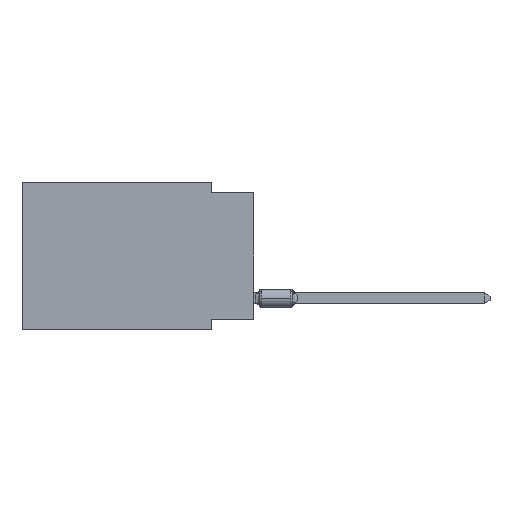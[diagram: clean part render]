
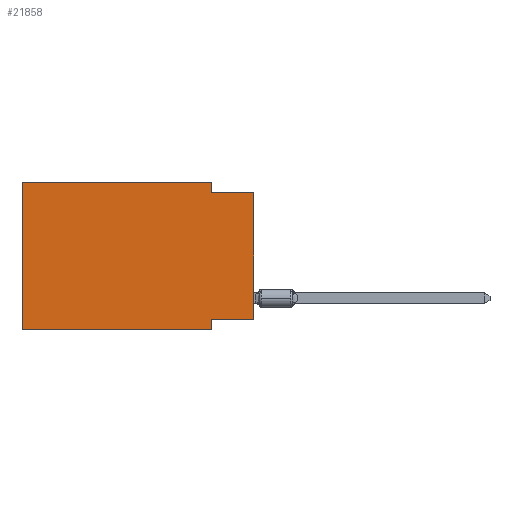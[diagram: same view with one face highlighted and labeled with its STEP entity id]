
A CAD part, left-side view. The second image highlights one B-rep face of the part: STEP entity #21858.
In plain terms, the highlighted planar face has unit normal (-1, 0, 0).
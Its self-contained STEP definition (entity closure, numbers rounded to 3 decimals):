
#670 = EDGE_LOOP ( 'NONE', ( #10321, #4042, #5680, #9196, #29071, #11287, #16565, #27068 ) ) ;
#789 = VECTOR ( 'NONE', #19286, 1000. ) ;
#1249 = CARTESIAN_POINT ( 'NONE',  ( 0., 2.54, -0.635 ) ) ;
#1926 = CARTESIAN_POINT ( 'NONE',  ( 0., 0., -0.635 ) ) ;
#3146 = CARTESIAN_POINT ( 'NONE',  ( 0., 0., 0. ) ) ;
#3660 = VECTOR ( 'NONE', #11100, 1000. ) ;
#4042 = ORIENTED_EDGE ( 'NONE', *, *, #23604, .F. ) ;
#4659 = VECTOR ( 'NONE', #29350, 1000. ) ;
#4697 = LINE ( 'NONE', #21197, #24072 ) ;
#5151 = VECTOR ( 'NONE', #9978, 1000. ) ;
#5238 = AXIS2_PLACEMENT_3D ( 'NONE', #20016, #29254, #8514 ) ;
#5680 = ORIENTED_EDGE ( 'NONE', *, *, #18365, .F. ) ;
#6106 = LINE ( 'NONE', #15334, #23554 ) ;
#7265 = DIRECTION ( 'NONE',  ( 0., 0., 1. ) ) ;
#7294 = VERTEX_POINT ( 'NONE', #9585 ) ;
#7629 = CARTESIAN_POINT ( 'NONE',  ( 0., 2.54, 0. ) ) ;
#7830 = VECTOR ( 'NONE', #20546, 1000. ) ;
#8514 = DIRECTION ( 'NONE',  ( 0., 0., -1. ) ) ;
#9196 = ORIENTED_EDGE ( 'NONE', *, *, #9801, .F. ) ;
#9410 = CARTESIAN_POINT ( 'NONE',  ( 0., 13.97, -8.89 ) ) ;
#9551 = DIRECTION ( 'NONE',  ( 0., 0., -1. ) ) ;
#9585 = CARTESIAN_POINT ( 'NONE',  ( 0., 2.54, -8.255 ) ) ;
#9686 = CARTESIAN_POINT ( 'NONE',  ( 0., 0., -0.635 ) ) ;
#9801 = EDGE_CURVE ( 'NONE', #24391, #15032, #28203, .T. ) ;
#9978 = DIRECTION ( 'NONE',  ( 0., -1., 0. ) ) ;
#10321 = ORIENTED_EDGE ( 'NONE', *, *, #23571, .T. ) ;
#11100 = DIRECTION ( 'NONE',  ( 0., -1., 0. ) ) ;
#11287 = ORIENTED_EDGE ( 'NONE', *, *, #15395, .T. ) ;
#11358 = EDGE_CURVE ( 'NONE', #7294, #27699, #4697, .T. ) ;
#13210 = CARTESIAN_POINT ( 'NONE',  ( 0., 13.97, -8.89 ) ) ;
#15032 = VERTEX_POINT ( 'NONE', #17481 ) ;
#15334 = CARTESIAN_POINT ( 'NONE',  ( 0., 13.97, 0. ) ) ;
#15395 = EDGE_CURVE ( 'NONE', #28291, #27699, #22596, .T. ) ;
#15564 = LINE ( 'NONE', #15872, #4659 ) ;
#15872 = CARTESIAN_POINT ( 'NONE',  ( 0., 0., -8.255 ) ) ;
#16565 = ORIENTED_EDGE ( 'NONE', *, *, #11358, .F. ) ;
#16592 = EDGE_CURVE ( 'NONE', #28291, #24391, #6106, .T. ) ;
#17481 = CARTESIAN_POINT ( 'NONE',  ( 0., 2.54, 0. ) ) ;
#17540 = VERTEX_POINT ( 'NONE', #1926 ) ;
#18365 = EDGE_CURVE ( 'NONE', #15032, #18476, #18839, .T. ) ;
#18418 = CARTESIAN_POINT ( 'NONE',  ( 0., 13.97, 0. ) ) ;
#18476 = VERTEX_POINT ( 'NONE', #1249 ) ;
#18556 = CARTESIAN_POINT ( 'NONE',  ( 0., 0., -8.255 ) ) ;
#18839 = LINE ( 'NONE', #7629, #789 ) ;
#19286 = DIRECTION ( 'NONE',  ( 0., 0., -1. ) ) ;
#19398 = EDGE_CURVE ( 'NONE', #19879, #7294, #15564, .T. ) ;
#19879 = VERTEX_POINT ( 'NONE', #18556 ) ;
#20016 = CARTESIAN_POINT ( 'NONE',  ( 0., 13.97, 0. ) ) ;
#20029 = DIRECTION ( 'NONE',  ( 0., 0., 1. ) ) ;
#20546 = DIRECTION ( 'NONE',  ( 0., -1., 0. ) ) ;
#21197 = CARTESIAN_POINT ( 'NONE',  ( 0., 2.54, -8.89 ) ) ;
#21858 = ADVANCED_FACE ( 'NONE', ( #26826 ), #22139, .F. ) ;
#21866 = CARTESIAN_POINT ( 'NONE',  ( 0., 2.54, -8.89 ) ) ;
#22139 = PLANE ( 'NONE',  #5238 ) ;
#22596 = LINE ( 'NONE', #13210, #3660 ) ;
#23554 = VECTOR ( 'NONE', #20029, 1000. ) ;
#23571 = EDGE_CURVE ( 'NONE', #19879, #17540, #27999, .T. ) ;
#23604 = EDGE_CURVE ( 'NONE', #18476, #17540, #26315, .T. ) ;
#24072 = VECTOR ( 'NONE', #9551, 1000. ) ;
#24391 = VERTEX_POINT ( 'NONE', #26512 ) ;
#26315 = LINE ( 'NONE', #9686, #5151 ) ;
#26512 = CARTESIAN_POINT ( 'NONE',  ( 0., 13.97, 0. ) ) ;
#26826 = FACE_OUTER_BOUND ( 'NONE', #670, .T. ) ;
#27068 = ORIENTED_EDGE ( 'NONE', *, *, #19398, .F. ) ;
#27699 = VERTEX_POINT ( 'NONE', #21866 ) ;
#27999 = LINE ( 'NONE', #3146, #29318 ) ;
#28203 = LINE ( 'NONE', #18418, #7830 ) ;
#28291 = VERTEX_POINT ( 'NONE', #9410 ) ;
#29071 = ORIENTED_EDGE ( 'NONE', *, *, #16592, .F. ) ;
#29254 = DIRECTION ( 'NONE',  ( 1., 0., 0. ) ) ;
#29318 = VECTOR ( 'NONE', #7265, 1000. ) ;
#29350 = DIRECTION ( 'NONE',  ( 0., 1., 0. ) ) ;
